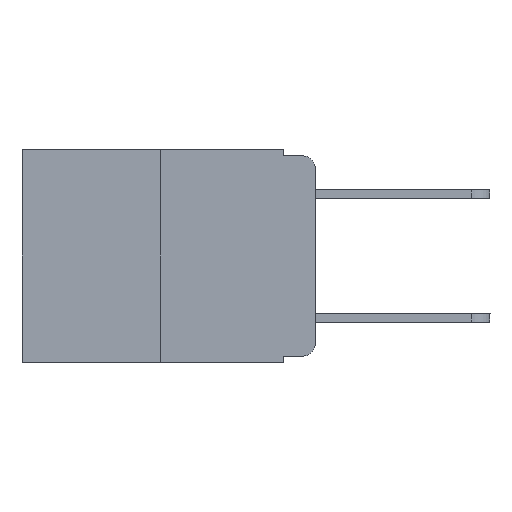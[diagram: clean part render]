
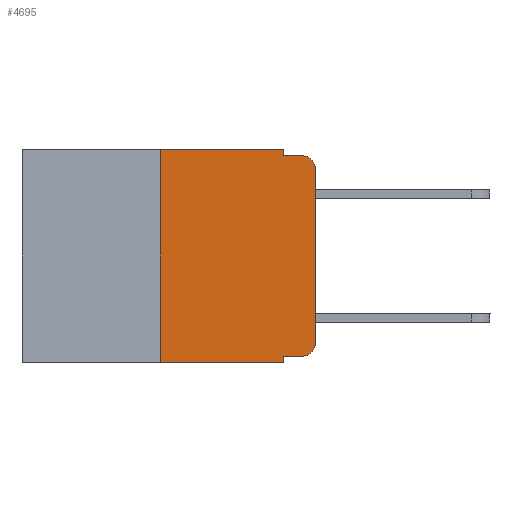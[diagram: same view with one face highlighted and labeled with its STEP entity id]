
A CAD part, left-side view. The second image highlights one B-rep face of the part: STEP entity #4695.
In plain terms, the highlighted planar face has unit normal (-1, 0, 0).
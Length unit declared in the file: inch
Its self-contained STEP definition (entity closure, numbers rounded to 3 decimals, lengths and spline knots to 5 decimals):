
#358 = VECTOR ( 'NONE', #16905, 39.37008 ) ;
#360 = EDGE_CURVE ( 'NONE', #3319, #1831, #14953, .T. ) ;
#753 = VECTOR ( 'NONE', #12880, 39.37008 ) ;
#938 = CARTESIAN_POINT ( 'NONE',  ( 0., 0.051, -0.01 ) ) ;
#1035 = CARTESIAN_POINT ( 'NONE',  ( 0., 0.25, 0. ) ) ;
#1049 = CARTESIAN_POINT ( 'NONE',  ( 0., 0.051, -0.01 ) ) ;
#1165 = DIRECTION ( 'NONE',  ( 0., 0., 1. ) ) ;
#1330 = CARTESIAN_POINT ( 'NONE',  ( 0., 0.473, -0.343 ) ) ;
#1537 = CARTESIAN_POINT ( 'NONE',  ( 0., 0.473, 0. ) ) ;
#1694 = ORIENTED_EDGE ( 'NONE', *, *, #14165, .F. ) ;
#1831 = VERTEX_POINT ( 'NONE', #13289 ) ;
#1989 = ORIENTED_EDGE ( 'NONE', *, *, #3493, .F. ) ;
#2078 = ORIENTED_EDGE ( 'NONE', *, *, #6112, .F. ) ;
#2213 = LINE ( 'NONE', #1035, #2436 ) ;
#2267 = DIRECTION ( 'NONE',  ( 1., 0., 0. ) ) ;
#2436 = VECTOR ( 'NONE', #1165, 39.37008 ) ;
#2518 = DIRECTION ( 'NONE',  ( 0., 0., -1. ) ) ;
#2815 = AXIS2_PLACEMENT_3D ( 'NONE', #15436, #12314, #6640 ) ;
#3102 = CARTESIAN_POINT ( 'NONE',  ( 0., 0.051, -0.333 ) ) ;
#3319 = VERTEX_POINT ( 'NONE', #15725 ) ;
#3349 = EDGE_CURVE ( 'NONE', #17004, #15148, #10673, .T. ) ;
#3379 = LINE ( 'NONE', #1537, #10682 ) ;
#3493 = EDGE_CURVE ( 'NONE', #5347, #17004, #16465, .T. ) ;
#4259 = VERTEX_POINT ( 'NONE', #9500 ) ;
#4656 = CARTESIAN_POINT ( 'NONE',  ( 0., 0.02, -0.03 ) ) ;
#4695 = ADVANCED_FACE ( 'NONE', ( #15572 ), #11648, .F. ) ;
#4938 = CARTESIAN_POINT ( 'NONE',  ( 0., 0.051, 0. ) ) ;
#5251 = DIRECTION ( 'NONE',  ( 0., -1., 0. ) ) ;
#5347 = VERTEX_POINT ( 'NONE', #4938 ) ;
#5524 = VECTOR ( 'NONE', #15034, 39.37008 ) ;
#5775 = ORIENTED_EDGE ( 'NONE', *, *, #17368, .T. ) ;
#6112 = EDGE_CURVE ( 'NONE', #3319, #7122, #2213, .T. ) ;
#6640 = DIRECTION ( 'NONE',  ( 0., 0., -1. ) ) ;
#7122 = VERTEX_POINT ( 'NONE', #18449 ) ;
#7194 = EDGE_CURVE ( 'NONE', #9865, #1831, #17541, .T. ) ;
#7601 = VERTEX_POINT ( 'NONE', #14364 ) ;
#8934 = LINE ( 'NONE', #3102, #5524 ) ;
#9097 = AXIS2_PLACEMENT_3D ( 'NONE', #11519, #2267, #2518 ) ;
#9284 = ORIENTED_EDGE ( 'NONE', *, *, #360, .T. ) ;
#9357 = EDGE_CURVE ( 'NONE', #9865, #7601, #8934, .T. ) ;
#9500 = CARTESIAN_POINT ( 'NONE',  ( 0., 0., -0.03 ) ) ;
#9839 = DIRECTION ( 'NONE',  ( 0., 0., -1. ) ) ;
#9865 = VERTEX_POINT ( 'NONE', #18119 ) ;
#10065 = EDGE_CURVE ( 'NONE', #7601, #12592, #18207, .T. ) ;
#10178 = LINE ( 'NONE', #10530, #11780 ) ;
#10317 = DIRECTION ( 'NONE',  ( 0., -1., 0. ) ) ;
#10530 = CARTESIAN_POINT ( 'NONE',  ( 0., 0., 0. ) ) ;
#10654 = DIRECTION ( 'NONE',  ( -1., 0., 0. ) ) ;
#10666 = VECTOR ( 'NONE', #9839, 39.37008 ) ;
#10673 = LINE ( 'NONE', #1049, #18766 ) ;
#10682 = VECTOR ( 'NONE', #10317, 39.37008 ) ;
#10971 = CIRCLE ( 'NONE', #11959, 0.02 ) ;
#11062 = CARTESIAN_POINT ( 'NONE',  ( 0., 0., -0.313 ) ) ;
#11519 = CARTESIAN_POINT ( 'NONE',  ( 0., 0.473, 0. ) ) ;
#11648 = PLANE ( 'NONE',  #9097 ) ;
#11780 = VECTOR ( 'NONE', #18131, 39.37008 ) ;
#11959 = AXIS2_PLACEMENT_3D ( 'NONE', #4656, #10654, #16613 ) ;
#12314 = DIRECTION ( 'NONE',  ( -1., 0., 0. ) ) ;
#12501 = ORIENTED_EDGE ( 'NONE', *, *, #7194, .F. ) ;
#12592 = VERTEX_POINT ( 'NONE', #11062 ) ;
#12612 = ORIENTED_EDGE ( 'NONE', *, *, #3349, .F. ) ;
#12880 = DIRECTION ( 'NONE',  ( 0., -1., 0. ) ) ;
#12913 = ORIENTED_EDGE ( 'NONE', *, *, #10065, .T. ) ;
#13289 = CARTESIAN_POINT ( 'NONE',  ( 0., 0.051, -0.343 ) ) ;
#14162 = CARTESIAN_POINT ( 'NONE',  ( 0., 0.02, -0.01 ) ) ;
#14165 = EDGE_CURVE ( 'NONE', #7122, #5347, #3379, .T. ) ;
#14364 = CARTESIAN_POINT ( 'NONE',  ( 0., 0.02, -0.333 ) ) ;
#14953 = LINE ( 'NONE', #1330, #753 ) ;
#15034 = DIRECTION ( 'NONE',  ( 0., -1., 0. ) ) ;
#15148 = VERTEX_POINT ( 'NONE', #14162 ) ;
#15427 = EDGE_CURVE ( 'NONE', #12592, #4259, #10178, .T. ) ;
#15436 = CARTESIAN_POINT ( 'NONE',  ( 0., 0.02, -0.313 ) ) ;
#15572 = FACE_OUTER_BOUND ( 'NONE', #16617, .T. ) ;
#15725 = CARTESIAN_POINT ( 'NONE',  ( 0., 0.25, -0.343 ) ) ;
#16465 = LINE ( 'NONE', #17440, #10666 ) ;
#16613 = DIRECTION ( 'NONE',  ( 0., 0., -1. ) ) ;
#16617 = EDGE_LOOP ( 'NONE', ( #17303, #5775, #12612, #1989, #1694, #2078, #9284, #12501, #18126, #12913 ) ) ;
#16905 = DIRECTION ( 'NONE',  ( 0., 0., -1. ) ) ;
#16975 = CARTESIAN_POINT ( 'NONE',  ( 0., 0.051, 0. ) ) ;
#17004 = VERTEX_POINT ( 'NONE', #938 ) ;
#17303 = ORIENTED_EDGE ( 'NONE', *, *, #15427, .T. ) ;
#17368 = EDGE_CURVE ( 'NONE', #4259, #15148, #10971, .T. ) ;
#17440 = CARTESIAN_POINT ( 'NONE',  ( 0., 0.051, 0. ) ) ;
#17541 = LINE ( 'NONE', #16975, #358 ) ;
#18119 = CARTESIAN_POINT ( 'NONE',  ( 0., 0.051, -0.333 ) ) ;
#18126 = ORIENTED_EDGE ( 'NONE', *, *, #9357, .T. ) ;
#18131 = DIRECTION ( 'NONE',  ( 0., 0., 1. ) ) ;
#18207 = CIRCLE ( 'NONE', #2815, 0.02 ) ;
#18449 = CARTESIAN_POINT ( 'NONE',  ( 0., 0.25, 0. ) ) ;
#18766 = VECTOR ( 'NONE', #5251, 39.37008 ) ;
